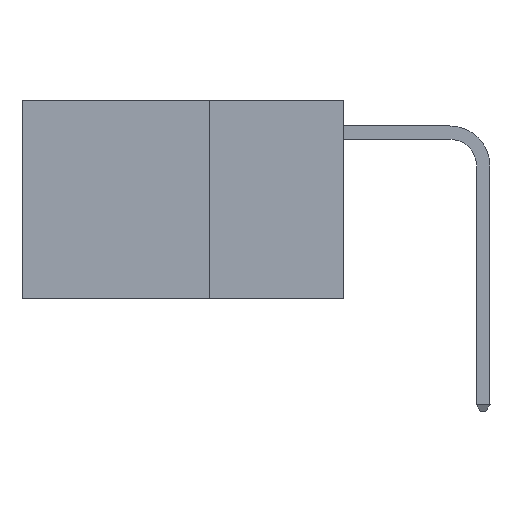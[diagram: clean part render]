
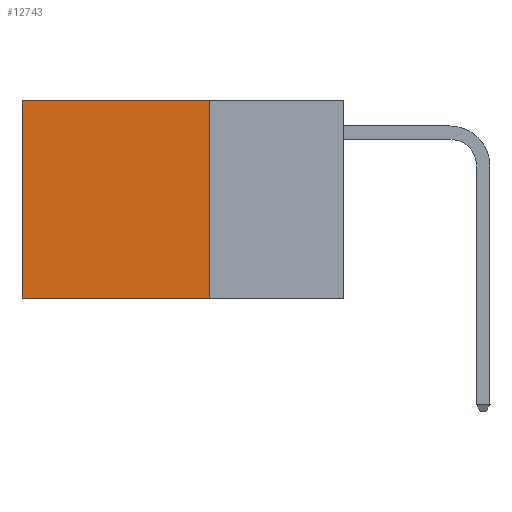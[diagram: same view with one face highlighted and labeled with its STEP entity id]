
A CAD part, left-side view. The second image highlights one B-rep face of the part: STEP entity #12743.
In plain terms, the highlighted planar face has unit normal (-1, 0, 0).
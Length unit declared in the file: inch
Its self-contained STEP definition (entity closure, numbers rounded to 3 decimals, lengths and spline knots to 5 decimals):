
#867 = EDGE_CURVE ( 'NONE', #9936, #6702, #10425, .T. ) ;
#1110 = VERTEX_POINT ( 'NONE', #8255 ) ;
#1240 = CARTESIAN_POINT ( 'NONE',  ( 0.2625, 0.25, -0.37 ) ) ;
#1516 = CARTESIAN_POINT ( 'NONE',  ( 0.2625, 0.25, 0. ) ) ;
#1993 = ORIENTED_EDGE ( 'NONE', *, *, #6871, .F. ) ;
#2339 = LINE ( 'NONE', #4213, #2601 ) ;
#2601 = VECTOR ( 'NONE', #4116, 39.37008 ) ;
#2874 = DIRECTION ( 'NONE',  ( 1., 0., 0. ) ) ;
#3547 = VECTOR ( 'NONE', #6694, 39.37008 ) ;
#3634 = LINE ( 'NONE', #6751, #3547 ) ;
#3864 = ORIENTED_EDGE ( 'NONE', *, *, #6617, .T. ) ;
#4116 = DIRECTION ( 'NONE',  ( 0., 0., -1. ) ) ;
#4213 = CARTESIAN_POINT ( 'NONE',  ( 0.2625, 0.25, 0. ) ) ;
#5828 = CARTESIAN_POINT ( 'NONE',  ( 0.2625, 0.6, -0.37 ) ) ;
#6617 = EDGE_CURVE ( 'NONE', #7755, #6702, #3634, .T. ) ;
#6694 = DIRECTION ( 'NONE',  ( 0., 0., -1. ) ) ;
#6702 = VERTEX_POINT ( 'NONE', #5828 ) ;
#6751 = CARTESIAN_POINT ( 'NONE',  ( 0.2625, 0.6, 0. ) ) ;
#6871 = EDGE_CURVE ( 'NONE', #1110, #9936, #2339, .T. ) ;
#7743 = EDGE_CURVE ( 'NONE', #1110, #7755, #9195, .T. ) ;
#7755 = VERTEX_POINT ( 'NONE', #8441 ) ;
#8255 = CARTESIAN_POINT ( 'NONE',  ( 0.2625, 0.25, 0. ) ) ;
#8441 = CARTESIAN_POINT ( 'NONE',  ( 0.2625, 0.6, 0. ) ) ;
#8717 = CARTESIAN_POINT ( 'NONE',  ( 0.2625, 0.25, 0. ) ) ;
#8829 = DIRECTION ( 'NONE',  ( 0., 1., 0. ) ) ;
#9195 = LINE ( 'NONE', #8717, #10228 ) ;
#9581 = PLANE ( 'NONE',  #10187 ) ;
#9609 = EDGE_LOOP ( 'NONE', ( #3864, #14341, #1993, #11810 ) ) ;
#9936 = VERTEX_POINT ( 'NONE', #1240 ) ;
#10187 = AXIS2_PLACEMENT_3D ( 'NONE', #1516, #2874, #12142 ) ;
#10228 = VECTOR ( 'NONE', #8829, 39.37008 ) ;
#10410 = VECTOR ( 'NONE', #11655, 39.37008 ) ;
#10425 = LINE ( 'NONE', #11793, #10410 ) ;
#11655 = DIRECTION ( 'NONE',  ( 0., 1., 0. ) ) ;
#11793 = CARTESIAN_POINT ( 'NONE',  ( 0.2625, 0.25, -0.37 ) ) ;
#11810 = ORIENTED_EDGE ( 'NONE', *, *, #7743, .T. ) ;
#12142 = DIRECTION ( 'NONE',  ( 0., 0., -1. ) ) ;
#12645 = FACE_OUTER_BOUND ( 'NONE', #9609, .T. ) ;
#12743 = ADVANCED_FACE ( 'NONE', ( #12645 ), #9581, .F. ) ;
#14341 = ORIENTED_EDGE ( 'NONE', *, *, #867, .F. ) ;
